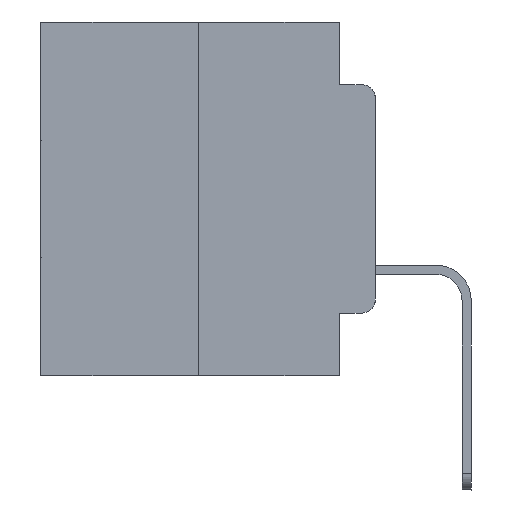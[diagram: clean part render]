
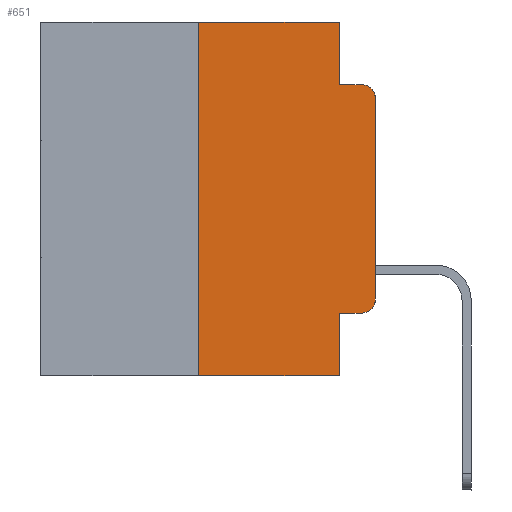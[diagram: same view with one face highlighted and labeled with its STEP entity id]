
A CAD part, left-side view. The second image highlights one B-rep face of the part: STEP entity #651.
In plain terms, the highlighted planar face has unit normal (-1, 0, 0).
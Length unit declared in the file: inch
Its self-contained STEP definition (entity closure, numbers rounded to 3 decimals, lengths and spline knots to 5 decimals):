
#175 = VECTOR ( 'NONE', #13712, 39.37008 ) ;
#651 = ADVANCED_FACE ( 'NONE', ( #14513 ), #24126, .F. ) ;
#1211 = CARTESIAN_POINT ( 'NONE',  ( 0., 0.051, 0. ) ) ;
#1714 = CARTESIAN_POINT ( 'NONE',  ( 0., 0.02, -0.3915 ) ) ;
#3274 = CARTESIAN_POINT ( 'NONE',  ( 0., 0.473, 0. ) ) ;
#3504 = VECTOR ( 'NONE', #11972, 39.37008 ) ;
#3707 = EDGE_CURVE ( 'NONE', #10173, #21072, #16711, .T. ) ;
#4259 = AXIS2_PLACEMENT_3D ( 'NONE', #3274, #7508, #7146 ) ;
#4280 = AXIS2_PLACEMENT_3D ( 'NONE', #1714, #16734, #6047 ) ;
#4427 = LINE ( 'NONE', #24096, #6413 ) ;
#4496 = CARTESIAN_POINT ( 'NONE',  ( 0., 0.02, -0.4115 ) ) ;
#6047 = DIRECTION ( 'NONE',  ( 0., 0., -1. ) ) ;
#6344 = CARTESIAN_POINT ( 'NONE',  ( 0., 0.051, -0.0885 ) ) ;
#6373 = VERTEX_POINT ( 'NONE', #9370 ) ;
#6413 = VECTOR ( 'NONE', #17885, 39.37008 ) ;
#6713 = VECTOR ( 'NONE', #16109, 39.37008 ) ;
#7146 = DIRECTION ( 'NONE',  ( 0., 0., -1. ) ) ;
#7445 = VECTOR ( 'NONE', #23392, 39.37008 ) ;
#7508 = DIRECTION ( 'NONE',  ( 1., 0., 0. ) ) ;
#7528 = DIRECTION ( 'NONE',  ( 0., 0., -1. ) ) ;
#8087 = VERTEX_POINT ( 'NONE', #26694 ) ;
#8180 = ORIENTED_EDGE ( 'NONE', *, *, #3707, .F. ) ;
#8252 = CARTESIAN_POINT ( 'NONE',  ( 0., 0.473, -0.5 ) ) ;
#8313 = CARTESIAN_POINT ( 'NONE',  ( 0., 0.051, -0.5 ) ) ;
#8534 = CARTESIAN_POINT ( 'NONE',  ( 0., 0.051, 0. ) ) ;
#9015 = CARTESIAN_POINT ( 'NONE',  ( 0., 0., -0.1085 ) ) ;
#9370 = CARTESIAN_POINT ( 'NONE',  ( 0., 0., -0.3915 ) ) ;
#10011 = DIRECTION ( 'NONE',  ( 0., -1., 0. ) ) ;
#10173 = VERTEX_POINT ( 'NONE', #12061 ) ;
#10219 = CARTESIAN_POINT ( 'NONE',  ( 0., 0.051, 0. ) ) ;
#10613 = EDGE_CURVE ( 'NONE', #26926, #10173, #21915, .T. ) ;
#10875 = VERTEX_POINT ( 'NONE', #4496 ) ;
#11657 = CARTESIAN_POINT ( 'NONE',  ( 0., 0.02, -0.1085 ) ) ;
#11972 = DIRECTION ( 'NONE',  ( 0., -1., 0. ) ) ;
#12029 = EDGE_CURVE ( 'NONE', #21072, #8087, #17897, .T. ) ;
#12061 = CARTESIAN_POINT ( 'NONE',  ( 0., 0.25, 0. ) ) ;
#12147 = VECTOR ( 'NONE', #10011, 39.37008 ) ;
#12236 = CARTESIAN_POINT ( 'NONE',  ( 0., 0.051, -0.4115 ) ) ;
#13268 = ORIENTED_EDGE ( 'NONE', *, *, #22577, .T. ) ;
#13365 = CARTESIAN_POINT ( 'NONE',  ( 0., 0.25, -0.5 ) ) ;
#13605 = VERTEX_POINT ( 'NONE', #12236 ) ;
#13712 = DIRECTION ( 'NONE',  ( 0., 0., 1. ) ) ;
#14130 = VERTEX_POINT ( 'NONE', #16104 ) ;
#14198 = LINE ( 'NONE', #8252, #26769 ) ;
#14513 = FACE_OUTER_BOUND ( 'NONE', #22683, .T. ) ;
#14525 = ORIENTED_EDGE ( 'NONE', *, *, #19164, .F. ) ;
#14626 = EDGE_CURVE ( 'NONE', #13605, #10875, #22093, .T. ) ;
#14922 = VERTEX_POINT ( 'NONE', #9015 ) ;
#15284 = ORIENTED_EDGE ( 'NONE', *, *, #10613, .F. ) ;
#15405 = ORIENTED_EDGE ( 'NONE', *, *, #14626, .T. ) ;
#15481 = CARTESIAN_POINT ( 'NONE',  ( 0., 0.25, 0. ) ) ;
#15727 = CIRCLE ( 'NONE', #4280, 0.02 ) ;
#16104 = CARTESIAN_POINT ( 'NONE',  ( 0., 0.02, -0.0885 ) ) ;
#16109 = DIRECTION ( 'NONE',  ( 0., 0., -1. ) ) ;
#16142 = CARTESIAN_POINT ( 'NONE',  ( 0., 0.473, 0. ) ) ;
#16627 = AXIS2_PLACEMENT_3D ( 'NONE', #11657, #26618, #7528 ) ;
#16711 = LINE ( 'NONE', #16142, #3504 ) ;
#16734 = DIRECTION ( 'NONE',  ( -1., 0., 0. ) ) ;
#16773 = EDGE_CURVE ( 'NONE', #8087, #14130, #21644, .T. ) ;
#17715 = ORIENTED_EDGE ( 'NONE', *, *, #19652, .T. ) ;
#17885 = DIRECTION ( 'NONE',  ( 0., 0., 1. ) ) ;
#17897 = LINE ( 'NONE', #1211, #6713 ) ;
#18128 = EDGE_CURVE ( 'NONE', #6373, #14922, #4427, .T. ) ;
#19164 = EDGE_CURVE ( 'NONE', #13605, #20317, #25825, .T. ) ;
#19652 = EDGE_CURVE ( 'NONE', #26926, #20317, #14198, .T. ) ;
#19690 = ORIENTED_EDGE ( 'NONE', *, *, #16773, .F. ) ;
#20317 = VERTEX_POINT ( 'NONE', #8313 ) ;
#20681 = ORIENTED_EDGE ( 'NONE', *, *, #18128, .T. ) ;
#20980 = DIRECTION ( 'NONE',  ( 0., -1., 0. ) ) ;
#21072 = VERTEX_POINT ( 'NONE', #8534 ) ;
#21397 = ORIENTED_EDGE ( 'NONE', *, *, #12029, .F. ) ;
#21644 = LINE ( 'NONE', #6344, #7445 ) ;
#21915 = LINE ( 'NONE', #15481, #175 ) ;
#22093 = LINE ( 'NONE', #26707, #12147 ) ;
#22497 = EDGE_CURVE ( 'NONE', #14922, #14130, #24026, .T. ) ;
#22577 = EDGE_CURVE ( 'NONE', #10875, #6373, #15727, .T. ) ;
#22683 = EDGE_LOOP ( 'NONE', ( #20681, #24991, #19690, #21397, #8180, #15284, #17715, #14525, #15405, #13268 ) ) ;
#22931 = DIRECTION ( 'NONE',  ( 0., 0., -1. ) ) ;
#23392 = DIRECTION ( 'NONE',  ( 0., -1., 0. ) ) ;
#24026 = CIRCLE ( 'NONE', #16627, 0.02 ) ;
#24096 = CARTESIAN_POINT ( 'NONE',  ( 0., 0., 0. ) ) ;
#24126 = PLANE ( 'NONE',  #4259 ) ;
#24991 = ORIENTED_EDGE ( 'NONE', *, *, #22497, .T. ) ;
#25158 = VECTOR ( 'NONE', #22931, 39.37008 ) ;
#25825 = LINE ( 'NONE', #10219, #25158 ) ;
#26618 = DIRECTION ( 'NONE',  ( -1., 0., 0. ) ) ;
#26694 = CARTESIAN_POINT ( 'NONE',  ( 0., 0.051, -0.0885 ) ) ;
#26707 = CARTESIAN_POINT ( 'NONE',  ( 0., 0.051, -0.4115 ) ) ;
#26769 = VECTOR ( 'NONE', #20980, 39.37008 ) ;
#26926 = VERTEX_POINT ( 'NONE', #13365 ) ;
